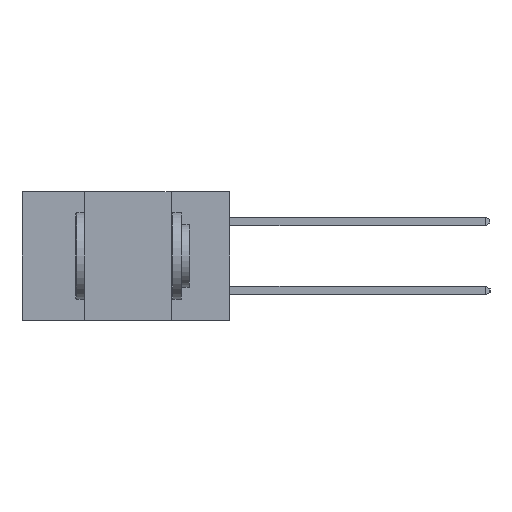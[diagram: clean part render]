
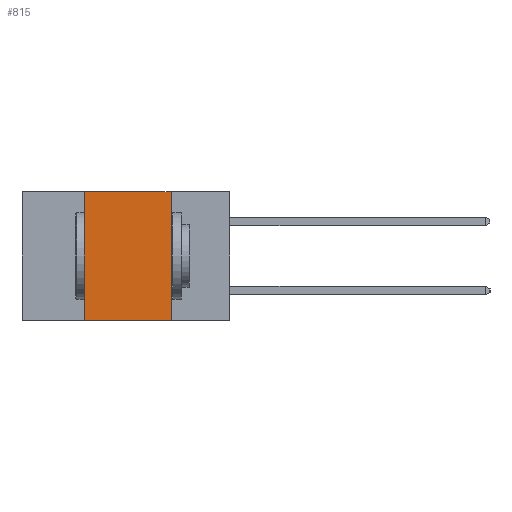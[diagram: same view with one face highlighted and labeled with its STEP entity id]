
A CAD part, left-side view. The second image highlights one B-rep face of the part: STEP entity #815.
In plain terms, the highlighted planar face has unit normal (-1, 0, 0).
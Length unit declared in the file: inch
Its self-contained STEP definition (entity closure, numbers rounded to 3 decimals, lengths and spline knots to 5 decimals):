
#218 = EDGE_CURVE ( 'NONE', #1802, #13214, #9318, .T. ) ;
#485 = CARTESIAN_POINT ( 'NONE',  ( 0., 0.42, -0.37 ) ) ;
#815 = ADVANCED_FACE ( 'NONE', ( #4910 ), #4948, .F. ) ;
#950 = AXIS2_PLACEMENT_3D ( 'NONE', #7729, #4898, #1440 ) ;
#981 = CARTESIAN_POINT ( 'NONE',  ( 0., 0.17, -0.37 ) ) ;
#1440 = DIRECTION ( 'NONE',  ( 0., 0., -1. ) ) ;
#1788 = EDGE_LOOP ( 'NONE', ( #7900, #7877, #13182, #8430 ) ) ;
#1802 = VERTEX_POINT ( 'NONE', #3047 ) ;
#3047 = CARTESIAN_POINT ( 'NONE',  ( 0., 0.17, 0. ) ) ;
#3144 = LINE ( 'NONE', #10417, #8723 ) ;
#4306 = VECTOR ( 'NONE', #4916, 39.37008 ) ;
#4624 = DIRECTION ( 'NONE',  ( 0., 0., -1. ) ) ;
#4803 = EDGE_CURVE ( 'NONE', #7982, #1802, #3144, .T. ) ;
#4877 = EDGE_CURVE ( 'NONE', #6821, #7982, #7295, .T. ) ;
#4898 = DIRECTION ( 'NONE',  ( 1., 0., 0. ) ) ;
#4910 = FACE_OUTER_BOUND ( 'NONE', #1788, .T. ) ;
#4916 = DIRECTION ( 'NONE',  ( 0., 0., 1. ) ) ;
#4948 = PLANE ( 'NONE',  #950 ) ;
#5507 = DIRECTION ( 'NONE',  ( 0., -1., 0. ) ) ;
#6319 = VECTOR ( 'NONE', #4624, 39.37008 ) ;
#6441 = CARTESIAN_POINT ( 'NONE',  ( 0., 0.6, -0.37 ) ) ;
#6821 = VERTEX_POINT ( 'NONE', #485 ) ;
#7295 = LINE ( 'NONE', #9831, #4306 ) ;
#7729 = CARTESIAN_POINT ( 'NONE',  ( 0., 0.6, 0. ) ) ;
#7877 = ORIENTED_EDGE ( 'NONE', *, *, #4803, .F. ) ;
#7900 = ORIENTED_EDGE ( 'NONE', *, *, #218, .F. ) ;
#7982 = VERTEX_POINT ( 'NONE', #9927 ) ;
#8430 = ORIENTED_EDGE ( 'NONE', *, *, #11859, .T. ) ;
#8723 = VECTOR ( 'NONE', #10552, 39.37008 ) ;
#9318 = LINE ( 'NONE', #981, #6319 ) ;
#9831 = CARTESIAN_POINT ( 'NONE',  ( 0., 0.42, -0.37 ) ) ;
#9896 = CARTESIAN_POINT ( 'NONE',  ( 0., 0.17, -0.37 ) ) ;
#9927 = CARTESIAN_POINT ( 'NONE',  ( 0., 0.42, 0. ) ) ;
#10417 = CARTESIAN_POINT ( 'NONE',  ( 0., 0.6, 0. ) ) ;
#10552 = DIRECTION ( 'NONE',  ( 0., -1., 0. ) ) ;
#10760 = LINE ( 'NONE', #6441, #13148 ) ;
#11859 = EDGE_CURVE ( 'NONE', #6821, #13214, #10760, .T. ) ;
#13148 = VECTOR ( 'NONE', #5507, 39.37008 ) ;
#13182 = ORIENTED_EDGE ( 'NONE', *, *, #4877, .F. ) ;
#13214 = VERTEX_POINT ( 'NONE', #9896 ) ;
